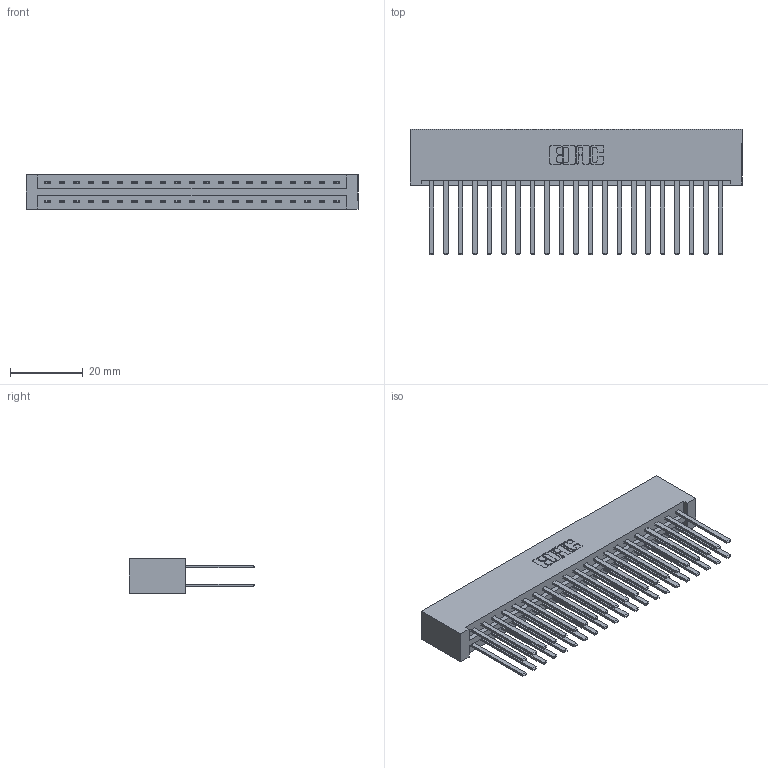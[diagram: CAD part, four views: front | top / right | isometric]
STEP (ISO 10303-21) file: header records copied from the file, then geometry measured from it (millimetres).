
FILE_DESCRIPTION (( 'STEP AP203' ), '1' );
FILE_NAME ('337-042-544-201.STEP', '2019-10-09T12:22:40', ( '' ), ( '' ), 'SwSTEP 2.0', 'SolidWorks 2016', '' );
FILE_SCHEMA (( 'CONFIG_CONTROL_DESIGN' ));
Length unit declared in the file: inch
Products named in the file (3): 337-042-544-201; 337 Part_No Mounting Lugs; 345-292-001_345-293-144
Assembly tree (43 placements, depth 2):
  337-042-544-201
    337 Part_No Mounting Lugs
    345-292-001_345-293-144  x42
Bounding box: 91.08 x 34.3 x 9.4 mm (x, y, z)
Volume: 10669.2 mm3; surface area: 13837 mm2
Topology: 43 solids, 43 shells, 2122 faces, 6293 edges, 4138 vertices
Faces by surface type: plane 1494, cylinder 628
Entity records: 18537 total; most frequent: CARTESIAN_POINT 3138, ORIENTED_EDGE 3074, DIRECTION 2697, EDGE_CURVE 1537, LINE 1421, VECTOR 1421, VERTEX_POINT 1022, AXIS2_PLACEMENT_3D 638
